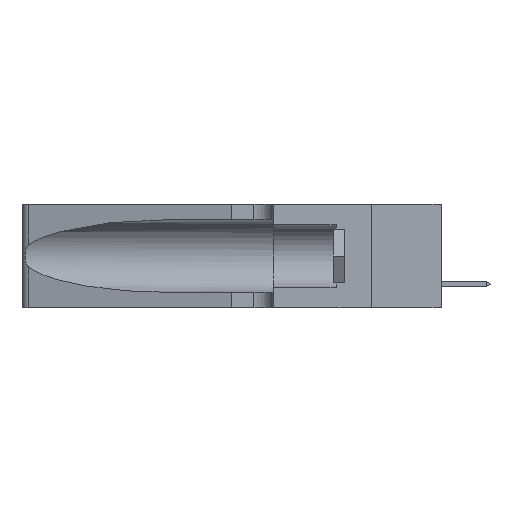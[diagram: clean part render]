
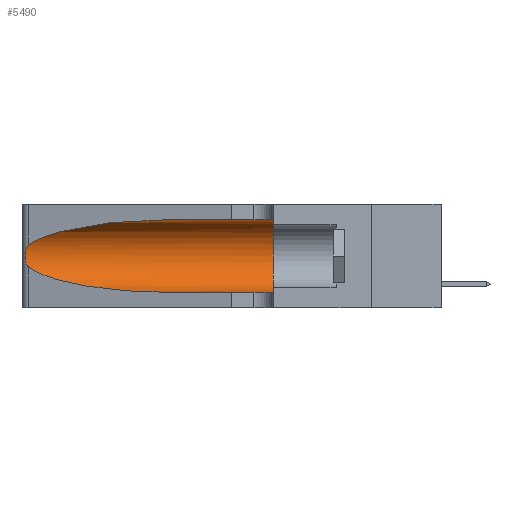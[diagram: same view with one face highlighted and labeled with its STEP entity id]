
A CAD part, left-side view. The second image highlights one B-rep face of the part: STEP entity #5490.
In plain terms, the highlighted cylindrical face has radius 3.308 mm (diameter 6.617 mm), a partial arc.
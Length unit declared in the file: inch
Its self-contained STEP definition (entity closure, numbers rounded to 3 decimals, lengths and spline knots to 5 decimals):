
#459 =( BOUNDED_CURVE ( )  B_SPLINE_CURVE ( 3, ( #34341, #17844, #1332, #6833 ),
 .UNSPECIFIED., .F., .T. ) 
 B_SPLINE_CURVE_WITH_KNOTS ( ( 4, 4 ),
 ( 1.5708, 2.84003 ),
 .UNSPECIFIED. ) 
 CURVE ( )  GEOMETRIC_REPRESENTATION_ITEM ( )  RATIONAL_B_SPLINE_CURVE ( ( 1., 0.87, 0.87, 1. ) ) 
 REPRESENTATION_ITEM ( '' )  );
#576 = ORIENTED_EDGE ( 'NONE', *, *, #11935, .F. ) ;
#1332 = CARTESIAN_POINT ( 'NONE',  ( 0.2373, 1.15595, 0.28018 ) ) ;
#1844 = ORIENTED_EDGE ( 'NONE', *, *, #9612, .T. ) ;
#2560 = CARTESIAN_POINT ( 'NONE',  ( 0.25789, 1.23486, 0.15765 ) ) ;
#2730 = ORIENTED_EDGE ( 'NONE', *, *, #31013, .T. ) ;
#4033 = B_SPLINE_CURVE_WITH_KNOTS ( 'NONE', 3,
 ( #18719, #21629, #4952, #32365, #13127, #10492, #27416, #29838, #13246, #16067, #2560, #5070, #24405, #7836 ),
 .UNSPECIFIED., .F., .F.,
 ( 4, 2, 2, 2, 2, 2, 4 ),
 ( 0., 0.00027, 0.00053, 0.00107, 0.0016, 0.00187, 0.00214 ),
 .UNSPECIFIED. ) ;
#4072 = EDGE_CURVE ( 'NONE', #22785, #30604, #4033, .T. ) ;
#4952 = CARTESIAN_POINT ( 'NONE',  ( 0.25639, 1.23184, 0.21858 ) ) ;
#5070 = CARTESIAN_POINT ( 'NONE',  ( 0.25639, 1.23186, 0.15144 ) ) ;
#5446 = DIRECTION ( 'NONE',  ( 0., 0., 1. ) ) ;
#5490 = ADVANCED_FACE ( 'NONE', ( #11810 ), #30412, .F. ) ;
#5963 = CARTESIAN_POINT ( 'NONE',  ( 0.25487, 1.22718, 0.22369 ) ) ;
#6204 = DIRECTION ( 'NONE',  ( 0., -1., 0. ) ) ;
#6820 =( BOUNDED_CURVE ( )  B_SPLINE_CURVE ( 3, ( #21558, #13547, #16471, #19490 ),
 .UNSPECIFIED., .F., .T. ) 
 B_SPLINE_CURVE_WITH_KNOTS ( ( 4, 4 ),
 ( 3.44316, 4.71239 ),
 .UNSPECIFIED. ) 
 CURVE ( )  GEOMETRIC_REPRESENTATION_ITEM ( )  RATIONAL_B_SPLINE_CURVE ( ( 1., 0.87, 0.87, 1. ) ) 
 REPRESENTATION_ITEM ( '' )  );
#6833 = CARTESIAN_POINT ( 'NONE',  ( 0.25487, 1.22718, 0.22369 ) ) ;
#7675 = ORIENTED_EDGE ( 'NONE', *, *, #27467, .T. ) ;
#7836 = CARTESIAN_POINT ( 'NONE',  ( 0.25487, 1.22718, 0.14631 ) ) ;
#9085 = DIRECTION ( 'NONE',  ( 0., -1., 0. ) ) ;
#9440 = LINE ( 'NONE', #26110, #34452 ) ;
#9612 = EDGE_CURVE ( 'NONE', #15352, #13219, #9440, .T. ) ;
#9698 = ORIENTED_EDGE ( 'NONE', *, *, #33532, .F. ) ;
#10492 = CARTESIAN_POINT ( 'NONE',  ( 0.26018, 1.23835, 0.19895 ) ) ;
#10703 = DIRECTION ( 'NONE',  ( 0., 0., -1. ) ) ;
#11810 = FACE_OUTER_BOUND ( 'NONE', #33380, .T. ) ;
#11935 = EDGE_CURVE ( 'NONE', #20299, #27493, #27889, .T. ) ;
#12933 = AXIS2_PLACEMENT_3D ( 'NONE', #19217, #24552, #5446 ) ;
#12983 = CARTESIAN_POINT ( 'NONE',  ( 0.1305, 1.61858, 0.185 ) ) ;
#13127 = CARTESIAN_POINT ( 'NONE',  ( 0.25854, 1.2359, 0.20912 ) ) ;
#13219 = VERTEX_POINT ( 'NONE', #22982 ) ;
#13246 = CARTESIAN_POINT ( 'NONE',  ( 0.26017, 1.23833, 0.17102 ) ) ;
#13547 = CARTESIAN_POINT ( 'NONE',  ( 0.2373, 1.15595, 0.08982 ) ) ;
#15352 = VERTEX_POINT ( 'NONE', #30811 ) ;
#16067 = CARTESIAN_POINT ( 'NONE',  ( 0.25856, 1.23593, 0.16098 ) ) ;
#16356 = CARTESIAN_POINT ( 'NONE',  ( 0.1305, 0.35, 0.31525 ) ) ;
#16471 = CARTESIAN_POINT ( 'NONE',  ( 0.18966, 0.96281, 0.05475 ) ) ;
#16565 = AXIS2_PLACEMENT_3D ( 'NONE', #12983, #27289, #10703 ) ;
#17844 = CARTESIAN_POINT ( 'NONE',  ( 0.18966, 0.96281, 0.31525 ) ) ;
#18719 = CARTESIAN_POINT ( 'NONE',  ( 0.25487, 1.22718, 0.22369 ) ) ;
#19217 = CARTESIAN_POINT ( 'NONE',  ( 0.1305, 0.35, 0.185 ) ) ;
#19490 = CARTESIAN_POINT ( 'NONE',  ( 0.1305, 0.72297, 0.05475 ) ) ;
#19938 = ORIENTED_EDGE ( 'NONE', *, *, #4072, .T. ) ;
#20299 = VERTEX_POINT ( 'NONE', #23040 ) ;
#21558 = CARTESIAN_POINT ( 'NONE',  ( 0.25487, 1.22718, 0.14631 ) ) ;
#21629 = CARTESIAN_POINT ( 'NONE',  ( 0.25555, 1.22994, 0.2215 ) ) ;
#22784 = CARTESIAN_POINT ( 'NONE',  ( 0.1305, 1.61858, 0.31525 ) ) ;
#22785 = VERTEX_POINT ( 'NONE', #5963 ) ;
#22982 = CARTESIAN_POINT ( 'NONE',  ( 0.1305, 0.35, 0.05475 ) ) ;
#23040 = CARTESIAN_POINT ( 'NONE',  ( 0.1305, 0.72297, 0.31525 ) ) ;
#24405 = CARTESIAN_POINT ( 'NONE',  ( 0.25555, 1.22993, 0.14849 ) ) ;
#24552 = DIRECTION ( 'NONE',  ( 0., 1., 0. ) ) ;
#26110 = CARTESIAN_POINT ( 'NONE',  ( 0.1305, 1.61858, 0.05475 ) ) ;
#27289 = DIRECTION ( 'NONE',  ( 0., -1., 0. ) ) ;
#27416 = CARTESIAN_POINT ( 'NONE',  ( 0.26075, 1.23896, 0.19203 ) ) ;
#27467 = EDGE_CURVE ( 'NONE', #30604, #15352, #6820, .T. ) ;
#27493 = VERTEX_POINT ( 'NONE', #16356 ) ;
#27889 = LINE ( 'NONE', #22784, #32619 ) ;
#29392 = CIRCLE ( 'NONE', #12933, 0.13025 ) ;
#29838 = CARTESIAN_POINT ( 'NONE',  ( 0.26075, 1.23896, 0.178 ) ) ;
#30412 = CYLINDRICAL_SURFACE ( 'NONE', #16565, 0.13025 ) ;
#30604 = VERTEX_POINT ( 'NONE', #35239 ) ;
#30811 = CARTESIAN_POINT ( 'NONE',  ( 0.1305, 0.72297, 0.05475 ) ) ;
#31013 = EDGE_CURVE ( 'NONE', #20299, #22785, #459, .T. ) ;
#32365 = CARTESIAN_POINT ( 'NONE',  ( 0.25787, 1.23484, 0.2124 ) ) ;
#32619 = VECTOR ( 'NONE', #6204, 39.37008 ) ;
#33380 = EDGE_LOOP ( 'NONE', ( #2730, #19938, #7675, #1844, #9698, #576 ) ) ;
#33532 = EDGE_CURVE ( 'NONE', #27493, #13219, #29392, .T. ) ;
#34341 = CARTESIAN_POINT ( 'NONE',  ( 0.1305, 0.72297, 0.31525 ) ) ;
#34452 = VECTOR ( 'NONE', #9085, 39.37008 ) ;
#35239 = CARTESIAN_POINT ( 'NONE',  ( 0.25487, 1.22718, 0.14631 ) ) ;
